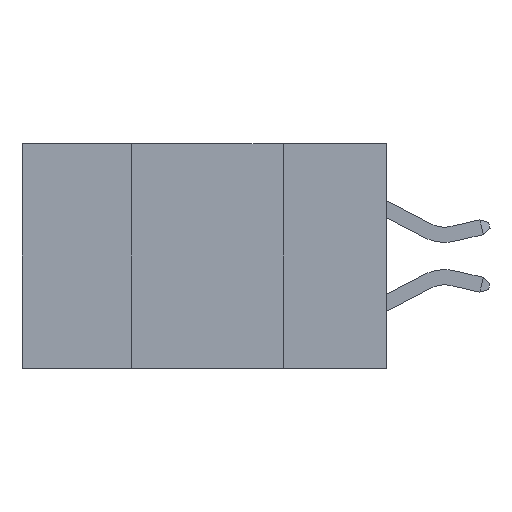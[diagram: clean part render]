
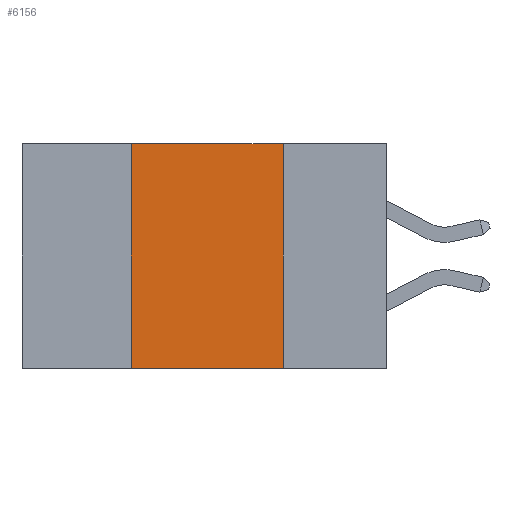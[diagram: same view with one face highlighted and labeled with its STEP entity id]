
A CAD part, left-side view. The second image highlights one B-rep face of the part: STEP entity #6156.
In plain terms, the highlighted planar face has unit normal (-1, 0, 0).
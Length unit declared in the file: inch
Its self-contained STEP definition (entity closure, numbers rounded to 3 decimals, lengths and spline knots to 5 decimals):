
#362 = LINE ( 'NONE', #3831, #10889 ) ;
#794 = VERTEX_POINT ( 'NONE', #8220 ) ;
#1516 = VECTOR ( 'NONE', #1992, 39.37008 ) ;
#1811 = DIRECTION ( 'NONE',  ( 0., -1., 0. ) ) ;
#1992 = DIRECTION ( 'NONE',  ( 0., -1., 0. ) ) ;
#3781 = VECTOR ( 'NONE', #8033, 39.37008 ) ;
#3831 = CARTESIAN_POINT ( 'NONE',  ( 0., 0.6, -0.37 ) ) ;
#6156 = ADVANCED_FACE ( 'NONE', ( #10064 ), #21903, .F. ) ;
#6350 = CARTESIAN_POINT ( 'NONE',  ( 0., 0.42, 0. ) ) ;
#6604 = CARTESIAN_POINT ( 'NONE',  ( 0., 0.42, -0.37 ) ) ;
#7145 = VERTEX_POINT ( 'NONE', #20042 ) ;
#7240 = ORIENTED_EDGE ( 'NONE', *, *, #9412, .F. ) ;
#7942 = CARTESIAN_POINT ( 'NONE',  ( 0., 0.17, 0. ) ) ;
#8002 = EDGE_CURVE ( 'NONE', #26947, #794, #362, .T. ) ;
#8033 = DIRECTION ( 'NONE',  ( 0., 0., -1. ) ) ;
#8220 = CARTESIAN_POINT ( 'NONE',  ( 0., 0.17, -0.37 ) ) ;
#8452 = DIRECTION ( 'NONE',  ( 0., 0., 1. ) ) ;
#8832 = LINE ( 'NONE', #6350, #19273 ) ;
#9406 = CARTESIAN_POINT ( 'NONE',  ( 0., 0.6, 0. ) ) ;
#9412 = EDGE_CURVE ( 'NONE', #26947, #24689, #8832, .T. ) ;
#10064 = FACE_OUTER_BOUND ( 'NONE', #20319, .T. ) ;
#10447 = ORIENTED_EDGE ( 'NONE', *, *, #8002, .T. ) ;
#10889 = VECTOR ( 'NONE', #1811, 39.37008 ) ;
#12230 = EDGE_CURVE ( 'NONE', #7145, #794, #20457, .T. ) ;
#12686 = LINE ( 'NONE', #20825, #1516 ) ;
#13649 = DIRECTION ( 'NONE',  ( 0., 0., -1. ) ) ;
#15801 = ORIENTED_EDGE ( 'NONE', *, *, #12230, .F. ) ;
#17048 = ORIENTED_EDGE ( 'NONE', *, *, #17668, .F. ) ;
#17668 = EDGE_CURVE ( 'NONE', #24689, #7145, #12686, .T. ) ;
#18653 = AXIS2_PLACEMENT_3D ( 'NONE', #9406, #26031, #13649 ) ;
#19273 = VECTOR ( 'NONE', #8452, 39.37008 ) ;
#20042 = CARTESIAN_POINT ( 'NONE',  ( 0., 0.17, 0. ) ) ;
#20319 = EDGE_LOOP ( 'NONE', ( #15801, #17048, #7240, #10447 ) ) ;
#20457 = LINE ( 'NONE', #7942, #3781 ) ;
#20825 = CARTESIAN_POINT ( 'NONE',  ( 0., 0.6, 0. ) ) ;
#21903 = PLANE ( 'NONE',  #18653 ) ;
#22122 = CARTESIAN_POINT ( 'NONE',  ( 0., 0.42, 0. ) ) ;
#24689 = VERTEX_POINT ( 'NONE', #22122 ) ;
#26031 = DIRECTION ( 'NONE',  ( 1., 0., 0. ) ) ;
#26947 = VERTEX_POINT ( 'NONE', #6604 ) ;
